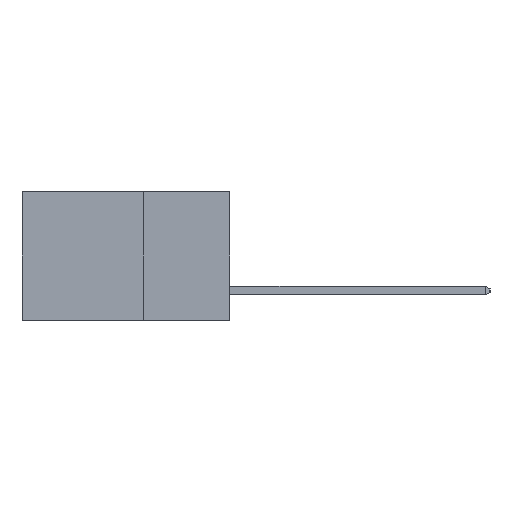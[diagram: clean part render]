
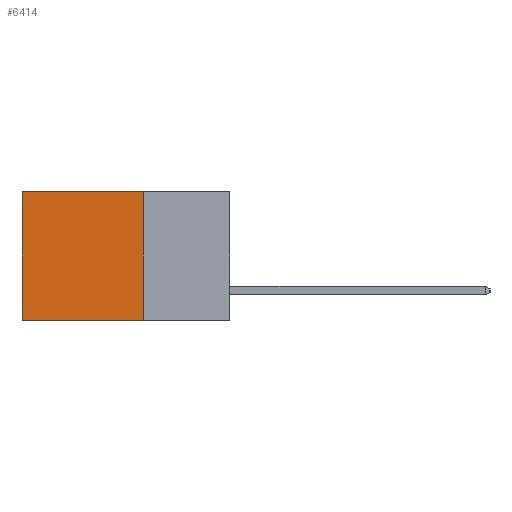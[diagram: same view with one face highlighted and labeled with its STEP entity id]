
A CAD part, left-side view. The second image highlights one B-rep face of the part: STEP entity #6414.
In plain terms, the highlighted planar face has unit normal (-1, 0, 0).
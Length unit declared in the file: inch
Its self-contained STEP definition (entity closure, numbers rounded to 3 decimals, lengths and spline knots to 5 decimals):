
#471 = DIRECTION ( 'NONE',  ( 0., 1., 0. ) ) ;
#781 = VECTOR ( 'NONE', #5305, 39.37008 ) ;
#1252 = DIRECTION ( 'NONE',  ( 0., 1., 0. ) ) ;
#1578 = CARTESIAN_POINT ( 'NONE',  ( 0.298, 0.25, -0.37 ) ) ;
#2675 = FACE_OUTER_BOUND ( 'NONE', #6930, .T. ) ;
#3043 = ORIENTED_EDGE ( 'NONE', *, *, #8476, .F. ) ;
#3255 = VERTEX_POINT ( 'NONE', #16437 ) ;
#3365 = CARTESIAN_POINT ( 'NONE',  ( 0.298, 0.25, 0. ) ) ;
#4433 = ORIENTED_EDGE ( 'NONE', *, *, #9033, .F. ) ;
#4614 = AXIS2_PLACEMENT_3D ( 'NONE', #21999, #18212, #6708 ) ;
#4651 = EDGE_CURVE ( 'NONE', #5770, #3255, #24003, .T. ) ;
#4728 = ORIENTED_EDGE ( 'NONE', *, *, #22469, .T. ) ;
#5305 = DIRECTION ( 'NONE',  ( 0., 0., -1. ) ) ;
#5386 = CARTESIAN_POINT ( 'NONE',  ( 0.298, 0.6, 0. ) ) ;
#5770 = VERTEX_POINT ( 'NONE', #5386 ) ;
#5885 = LINE ( 'NONE', #3365, #781 ) ;
#6414 = ADVANCED_FACE ( 'NONE', ( #2675 ), #16312, .F. ) ;
#6708 = DIRECTION ( 'NONE',  ( 0., 0., -1. ) ) ;
#6930 = EDGE_LOOP ( 'NONE', ( #16638, #4433, #3043, #4728 ) ) ;
#7171 = DIRECTION ( 'NONE',  ( 0., 0., -1. ) ) ;
#8222 = CARTESIAN_POINT ( 'NONE',  ( 0.298, 0.6, 0. ) ) ;
#8476 = EDGE_CURVE ( 'NONE', #22671, #21630, #5885, .T. ) ;
#9033 = EDGE_CURVE ( 'NONE', #21630, #3255, #22706, .T. ) ;
#10838 = CARTESIAN_POINT ( 'NONE',  ( 0.298, 0.25, -0.37 ) ) ;
#16312 = PLANE ( 'NONE',  #4614 ) ;
#16437 = CARTESIAN_POINT ( 'NONE',  ( 0.298, 0.6, -0.37 ) ) ;
#16638 = ORIENTED_EDGE ( 'NONE', *, *, #4651, .T. ) ;
#18212 = DIRECTION ( 'NONE',  ( 1., 0., 0. ) ) ;
#18904 = VECTOR ( 'NONE', #7171, 39.37008 ) ;
#20259 = VECTOR ( 'NONE', #471, 39.37008 ) ;
#20816 = CARTESIAN_POINT ( 'NONE',  ( 0.298, 0.25, 0. ) ) ;
#20844 = LINE ( 'NONE', #23509, #20259 ) ;
#21630 = VERTEX_POINT ( 'NONE', #1578 ) ;
#21999 = CARTESIAN_POINT ( 'NONE',  ( 0.298, 0.25, 0. ) ) ;
#22102 = VECTOR ( 'NONE', #1252, 39.37008 ) ;
#22469 = EDGE_CURVE ( 'NONE', #22671, #5770, #20844, .T. ) ;
#22671 = VERTEX_POINT ( 'NONE', #20816 ) ;
#22706 = LINE ( 'NONE', #10838, #22102 ) ;
#23509 = CARTESIAN_POINT ( 'NONE',  ( 0.298, 0.25, 0. ) ) ;
#24003 = LINE ( 'NONE', #8222, #18904 ) ;
